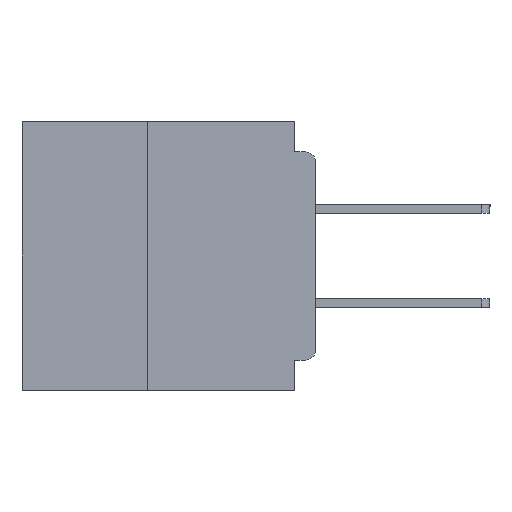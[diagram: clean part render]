
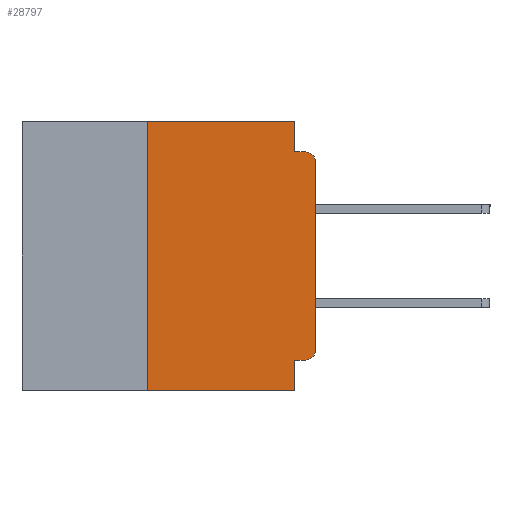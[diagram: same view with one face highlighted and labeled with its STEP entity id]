
A CAD part, left-side view. The second image highlights one B-rep face of the part: STEP entity #28797.
In plain terms, the highlighted planar face has unit normal (-1, 0, 0).
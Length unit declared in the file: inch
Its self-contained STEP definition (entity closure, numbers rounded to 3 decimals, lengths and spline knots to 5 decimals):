
#63 = ORIENTED_EDGE ( 'NONE', *, *, #46903, .F. ) ;
#492 = VERTEX_POINT ( 'NONE', #24439 ) ;
#639 = DIRECTION ( 'NONE',  ( 0., 0., -1. ) ) ;
#1075 = ORIENTED_EDGE ( 'NONE', *, *, #18590, .T. ) ;
#1345 = VERTEX_POINT ( 'NONE', #48010 ) ;
#2396 = ORIENTED_EDGE ( 'NONE', *, *, #7254, .F. ) ;
#3196 = VERTEX_POINT ( 'NONE', #34247 ) ;
#3749 = VECTOR ( 'NONE', #36536, 39.37008 ) ;
#4974 = VECTOR ( 'NONE', #639, 39.37008 ) ;
#6448 = DIRECTION ( 'NONE',  ( 0., -1., 0. ) ) ;
#7254 = EDGE_CURVE ( 'NONE', #10916, #19948, #38153, .T. ) ;
#8419 = CARTESIAN_POINT ( 'NONE',  ( 0., 0.031, 0. ) ) ;
#9061 = CARTESIAN_POINT ( 'NONE',  ( 0., 0.437, -0.4 ) ) ;
#9242 = ORIENTED_EDGE ( 'NONE', *, *, #12896, .F. ) ;
#9510 = CARTESIAN_POINT ( 'NONE',  ( 0., 0.015, -0.355 ) ) ;
#9591 = PLANE ( 'NONE',  #31491 ) ;
#10802 = CARTESIAN_POINT ( 'NONE',  ( 0., 0., 0. ) ) ;
#10916 = VERTEX_POINT ( 'NONE', #9510 ) ;
#12110 = DIRECTION ( 'NONE',  ( -1., 0., 0. ) ) ;
#12595 = ORIENTED_EDGE ( 'NONE', *, *, #50786, .T. ) ;
#12896 = EDGE_CURVE ( 'NONE', #3196, #13489, #25917, .T. ) ;
#13489 = VERTEX_POINT ( 'NONE', #20078 ) ;
#13951 = CARTESIAN_POINT ( 'NONE',  ( 0., 0.031, -0.355 ) ) ;
#14743 = LINE ( 'NONE', #10802, #26392 ) ;
#14808 = DIRECTION ( 'NONE',  ( 0., 0., 1. ) ) ;
#16221 = VERTEX_POINT ( 'NONE', #25469 ) ;
#17100 = LINE ( 'NONE', #18514, #44622 ) ;
#17549 = DIRECTION ( 'NONE',  ( 0., 0., -1. ) ) ;
#18203 = CARTESIAN_POINT ( 'NONE',  ( 0., 0.437, 0. ) ) ;
#18514 = CARTESIAN_POINT ( 'NONE',  ( 0., 0.031, -0.4 ) ) ;
#18590 = EDGE_CURVE ( 'NONE', #16221, #39759, #33893, .T. ) ;
#19491 = LINE ( 'NONE', #31724, #49393 ) ;
#19719 = CARTESIAN_POINT ( 'NONE',  ( 0., 0.25, -0.4 ) ) ;
#19946 = DIRECTION ( 'NONE',  ( -1., 0., 0. ) ) ;
#19948 = VERTEX_POINT ( 'NONE', #13951 ) ;
#19957 = CIRCLE ( 'NONE', #41212, 0.015 ) ;
#19979 = LINE ( 'NONE', #19719, #39595 ) ;
#20078 = CARTESIAN_POINT ( 'NONE',  ( 0., 0.031, -0.045 ) ) ;
#21317 = CARTESIAN_POINT ( 'NONE',  ( 0., 0.437, 0. ) ) ;
#22040 = ORIENTED_EDGE ( 'NONE', *, *, #36442, .T. ) ;
#23508 = CARTESIAN_POINT ( 'NONE',  ( 0., 0., -0.355 ) ) ;
#23644 = DIRECTION ( 'NONE',  ( 0., 0., 1. ) ) ;
#24439 = CARTESIAN_POINT ( 'NONE',  ( 0., 0., -0.06 ) ) ;
#24553 = EDGE_CURVE ( 'NONE', #19948, #39759, #17100, .T. ) ;
#25469 = CARTESIAN_POINT ( 'NONE',  ( 0., 0.25, -0.4 ) ) ;
#25917 = LINE ( 'NONE', #8419, #4974 ) ;
#26392 = VECTOR ( 'NONE', #14808, 39.37008 ) ;
#26507 = VECTOR ( 'NONE', #43043, 39.37008 ) ;
#26995 = ORIENTED_EDGE ( 'NONE', *, *, #48570, .F. ) ;
#27202 = CARTESIAN_POINT ( 'NONE',  ( 0., 0.25, 0. ) ) ;
#27882 = CARTESIAN_POINT ( 'NONE',  ( 0., 0.031, -0.4 ) ) ;
#28797 = ADVANCED_FACE ( 'NONE', ( #33870 ), #9591, .F. ) ;
#30246 = VERTEX_POINT ( 'NONE', #27202 ) ;
#31491 = AXIS2_PLACEMENT_3D ( 'NONE', #21317, #41012, #17549 ) ;
#31724 = CARTESIAN_POINT ( 'NONE',  ( 0., 0., -0.045 ) ) ;
#33748 = ORIENTED_EDGE ( 'NONE', *, *, #24553, .F. ) ;
#33870 = FACE_OUTER_BOUND ( 'NONE', #39463, .T. ) ;
#33893 = LINE ( 'NONE', #9061, #3749 ) ;
#34247 = CARTESIAN_POINT ( 'NONE',  ( 0., 0.031, 0. ) ) ;
#34277 = DIRECTION ( 'NONE',  ( 0., 0., -1. ) ) ;
#34353 = ORIENTED_EDGE ( 'NONE', *, *, #48334, .F. ) ;
#35229 = VERTEX_POINT ( 'NONE', #42603 ) ;
#35649 = CARTESIAN_POINT ( 'NONE',  ( 0., 0.015, -0.34 ) ) ;
#35652 = DIRECTION ( 'NONE',  ( 0., -1., 0. ) ) ;
#36442 = EDGE_CURVE ( 'NONE', #492, #1345, #19957, .T. ) ;
#36536 = DIRECTION ( 'NONE',  ( 0., -1., 0. ) ) ;
#38148 = EDGE_CURVE ( 'NONE', #35229, #492, #14743, .T. ) ;
#38153 = LINE ( 'NONE', #23508, #26507 ) ;
#39463 = EDGE_LOOP ( 'NONE', ( #46234, #22040, #63, #9242, #34353, #26995, #1075, #33748, #2396, #12595 ) ) ;
#39591 = DIRECTION ( 'NONE',  ( 0., 0., -1. ) ) ;
#39595 = VECTOR ( 'NONE', #23644, 39.37008 ) ;
#39759 = VERTEX_POINT ( 'NONE', #27882 ) ;
#40770 = LINE ( 'NONE', #18203, #49853 ) ;
#41012 = DIRECTION ( 'NONE',  ( 1., 0., 0. ) ) ;
#41212 = AXIS2_PLACEMENT_3D ( 'NONE', #43403, #19946, #47299 ) ;
#42603 = CARTESIAN_POINT ( 'NONE',  ( 0., 0., -0.34 ) ) ;
#43043 = DIRECTION ( 'NONE',  ( 0., 1., 0. ) ) ;
#43403 = CARTESIAN_POINT ( 'NONE',  ( 0., 0.015, -0.06 ) ) ;
#44622 = VECTOR ( 'NONE', #34277, 39.37008 ) ;
#46234 = ORIENTED_EDGE ( 'NONE', *, *, #38148, .T. ) ;
#46903 = EDGE_CURVE ( 'NONE', #13489, #1345, #19491, .T. ) ;
#47299 = DIRECTION ( 'NONE',  ( 0., 0., -1. ) ) ;
#48010 = CARTESIAN_POINT ( 'NONE',  ( 0., 0.015, -0.045 ) ) ;
#48334 = EDGE_CURVE ( 'NONE', #30246, #3196, #40770, .T. ) ;
#48570 = EDGE_CURVE ( 'NONE', #16221, #30246, #19979, .T. ) ;
#48769 = AXIS2_PLACEMENT_3D ( 'NONE', #35649, #12110, #39591 ) ;
#49218 = CIRCLE ( 'NONE', #48769, 0.015 ) ;
#49393 = VECTOR ( 'NONE', #35652, 39.37008 ) ;
#49853 = VECTOR ( 'NONE', #6448, 39.37008 ) ;
#50786 = EDGE_CURVE ( 'NONE', #10916, #35229, #49218, .T. ) ;
